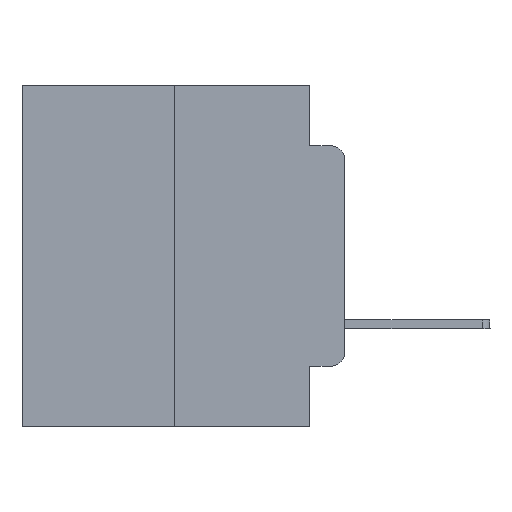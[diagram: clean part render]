
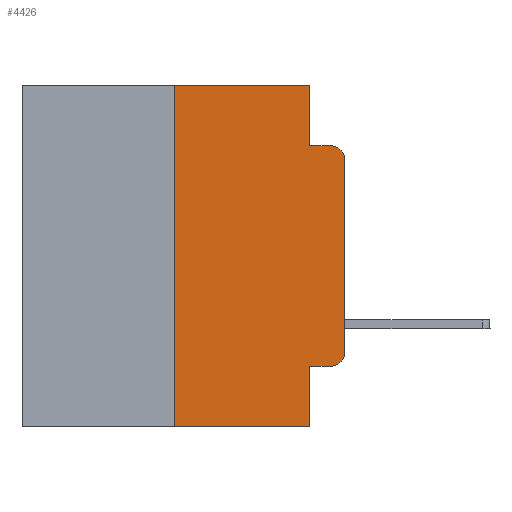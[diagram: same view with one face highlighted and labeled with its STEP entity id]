
A CAD part, left-side view. The second image highlights one B-rep face of the part: STEP entity #4426.
In plain terms, the highlighted planar face has unit normal (-1, 0, 0).
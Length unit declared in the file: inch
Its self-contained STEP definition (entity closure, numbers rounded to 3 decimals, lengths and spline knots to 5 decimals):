
#73 = DIRECTION ( 'NONE',  ( -1., 0., 0. ) ) ;
#810 = EDGE_CURVE ( 'NONE', #24126, #18860, #12160, .T. ) ;
#1177 = VERTEX_POINT ( 'NONE', #12249 ) ;
#2049 = VECTOR ( 'NONE', #24945, 39.37008 ) ;
#2183 = AXIS2_PLACEMENT_3D ( 'NONE', #3139, #5229, #11245 ) ;
#2216 = EDGE_CURVE ( 'NONE', #14907, #3242, #2558, .T. ) ;
#2288 = LINE ( 'NONE', #18921, #22175 ) ;
#2558 = CIRCLE ( 'NONE', #18557, 0.02 ) ;
#2672 = EDGE_CURVE ( 'NONE', #8083, #5037, #18317, .T. ) ;
#2850 = DIRECTION ( 'NONE',  ( 0., -1., 0. ) ) ;
#2901 = FACE_OUTER_BOUND ( 'NONE', #9662, .T. ) ;
#3132 = DIRECTION ( 'NONE',  ( 0., 0., -1. ) ) ;
#3139 = CARTESIAN_POINT ( 'NONE',  ( 0., 0.02, -0.1085 ) ) ;
#3242 = VERTEX_POINT ( 'NONE', #14969 ) ;
#3399 = ORIENTED_EDGE ( 'NONE', *, *, #16472, .F. ) ;
#3490 = DIRECTION ( 'NONE',  ( 0., 0., 1. ) ) ;
#3570 = VERTEX_POINT ( 'NONE', #22338 ) ;
#4076 = CARTESIAN_POINT ( 'NONE',  ( 0., 0.473, -0.5 ) ) ;
#4116 = VECTOR ( 'NONE', #3490, 39.37008 ) ;
#4426 = ADVANCED_FACE ( 'NONE', ( #2901 ), #15062, .F. ) ;
#4529 = VECTOR ( 'NONE', #2850, 39.37008 ) ;
#4629 = LINE ( 'NONE', #16492, #8720 ) ;
#4790 = CARTESIAN_POINT ( 'NONE',  ( 0., 0.051, -0.4115 ) ) ;
#5037 = VERTEX_POINT ( 'NONE', #11068 ) ;
#5188 = CARTESIAN_POINT ( 'NONE',  ( 0., 0.02, -0.4115 ) ) ;
#5229 = DIRECTION ( 'NONE',  ( -1., 0., 0. ) ) ;
#6066 = ORIENTED_EDGE ( 'NONE', *, *, #20279, .F. ) ;
#6147 = CARTESIAN_POINT ( 'NONE',  ( 0., 0.02, -0.0885 ) ) ;
#6150 = VERTEX_POINT ( 'NONE', #20478 ) ;
#7990 = DIRECTION ( 'NONE',  ( 0., 0., -1. ) ) ;
#8083 = VERTEX_POINT ( 'NONE', #23881 ) ;
#8199 = LINE ( 'NONE', #23320, #4116 ) ;
#8720 = VECTOR ( 'NONE', #25123, 39.37008 ) ;
#9371 = EDGE_CURVE ( 'NONE', #8083, #1177, #15287, .T. ) ;
#9662 = EDGE_LOOP ( 'NONE', ( #10186, #18352, #6066, #16324, #3399, #11787, #20338, #18956, #12512, #15058 ) ) ;
#10134 = EDGE_CURVE ( 'NONE', #6150, #18456, #15425, .T. ) ;
#10186 = ORIENTED_EDGE ( 'NONE', *, *, #16012, .T. ) ;
#11068 = CARTESIAN_POINT ( 'NONE',  ( 0., 0.051, -0.5 ) ) ;
#11245 = DIRECTION ( 'NONE',  ( 0., 0., -1. ) ) ;
#11787 = ORIENTED_EDGE ( 'NONE', *, *, #9371, .F. ) ;
#12160 = CIRCLE ( 'NONE', #2183, 0.02 ) ;
#12249 = CARTESIAN_POINT ( 'NONE',  ( 0., 0.25, 0. ) ) ;
#12512 = ORIENTED_EDGE ( 'NONE', *, *, #21854, .T. ) ;
#12741 = LINE ( 'NONE', #20919, #21256 ) ;
#14871 = VECTOR ( 'NONE', #22312, 39.37008 ) ;
#14889 = CARTESIAN_POINT ( 'NONE',  ( 0., 0.473, 0. ) ) ;
#14907 = VERTEX_POINT ( 'NONE', #5188 ) ;
#14969 = CARTESIAN_POINT ( 'NONE',  ( 0., 0., -0.3915 ) ) ;
#15058 = ORIENTED_EDGE ( 'NONE', *, *, #2216, .T. ) ;
#15062 = PLANE ( 'NONE',  #25878 ) ;
#15287 = LINE ( 'NONE', #17090, #2049 ) ;
#15425 = LINE ( 'NONE', #19405, #18832 ) ;
#16012 = EDGE_CURVE ( 'NONE', #3242, #24126, #8199, .T. ) ;
#16324 = ORIENTED_EDGE ( 'NONE', *, *, #10134, .F. ) ;
#16472 = EDGE_CURVE ( 'NONE', #1177, #6150, #12741, .T. ) ;
#16492 = CARTESIAN_POINT ( 'NONE',  ( 0., 0.051, -0.0885 ) ) ;
#16827 = DIRECTION ( 'NONE',  ( 0., 0., -1. ) ) ;
#17090 = CARTESIAN_POINT ( 'NONE',  ( 0., 0.25, 0. ) ) ;
#17772 = LINE ( 'NONE', #4790, #4529 ) ;
#18317 = LINE ( 'NONE', #4076, #14871 ) ;
#18352 = ORIENTED_EDGE ( 'NONE', *, *, #810, .T. ) ;
#18456 = VERTEX_POINT ( 'NONE', #20649 ) ;
#18557 = AXIS2_PLACEMENT_3D ( 'NONE', #23944, #73, #7990 ) ;
#18832 = VECTOR ( 'NONE', #3132, 39.37008 ) ;
#18860 = VERTEX_POINT ( 'NONE', #6147 ) ;
#18921 = CARTESIAN_POINT ( 'NONE',  ( 0., 0.051, 0. ) ) ;
#18956 = ORIENTED_EDGE ( 'NONE', *, *, #22566, .F. ) ;
#19405 = CARTESIAN_POINT ( 'NONE',  ( 0., 0.051, 0. ) ) ;
#20279 = EDGE_CURVE ( 'NONE', #18456, #18860, #4629, .T. ) ;
#20338 = ORIENTED_EDGE ( 'NONE', *, *, #2672, .T. ) ;
#20478 = CARTESIAN_POINT ( 'NONE',  ( 0., 0.051, 0. ) ) ;
#20649 = CARTESIAN_POINT ( 'NONE',  ( 0., 0.051, -0.0885 ) ) ;
#20919 = CARTESIAN_POINT ( 'NONE',  ( 0., 0.473, 0. ) ) ;
#21256 = VECTOR ( 'NONE', #22928, 39.37008 ) ;
#21854 = EDGE_CURVE ( 'NONE', #3570, #14907, #17772, .T. ) ;
#22175 = VECTOR ( 'NONE', #16827, 39.37008 ) ;
#22312 = DIRECTION ( 'NONE',  ( 0., -1., 0. ) ) ;
#22338 = CARTESIAN_POINT ( 'NONE',  ( 0., 0.051, -0.4115 ) ) ;
#22539 = CARTESIAN_POINT ( 'NONE',  ( 0., 0., -0.1085 ) ) ;
#22566 = EDGE_CURVE ( 'NONE', #3570, #5037, #2288, .T. ) ;
#22928 = DIRECTION ( 'NONE',  ( 0., -1., 0. ) ) ;
#22979 = DIRECTION ( 'NONE',  ( 1., 0., 0. ) ) ;
#23320 = CARTESIAN_POINT ( 'NONE',  ( 0., 0., 0. ) ) ;
#23881 = CARTESIAN_POINT ( 'NONE',  ( 0., 0.25, -0.5 ) ) ;
#23944 = CARTESIAN_POINT ( 'NONE',  ( 0., 0.02, -0.3915 ) ) ;
#24126 = VERTEX_POINT ( 'NONE', #22539 ) ;
#24945 = DIRECTION ( 'NONE',  ( 0., 0., 1. ) ) ;
#24996 = DIRECTION ( 'NONE',  ( 0., 0., -1. ) ) ;
#25123 = DIRECTION ( 'NONE',  ( 0., -1., 0. ) ) ;
#25878 = AXIS2_PLACEMENT_3D ( 'NONE', #14889, #22979, #24996 ) ;
